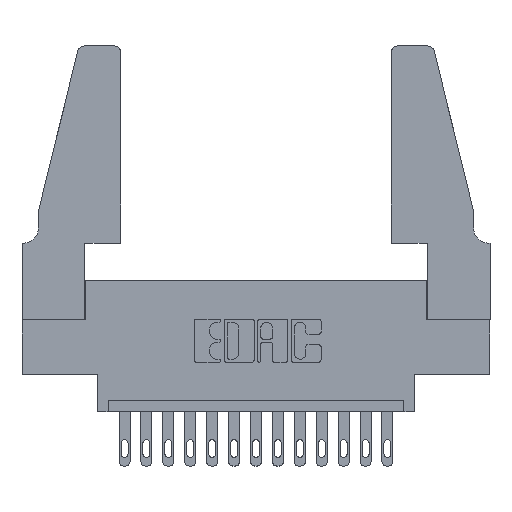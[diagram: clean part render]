
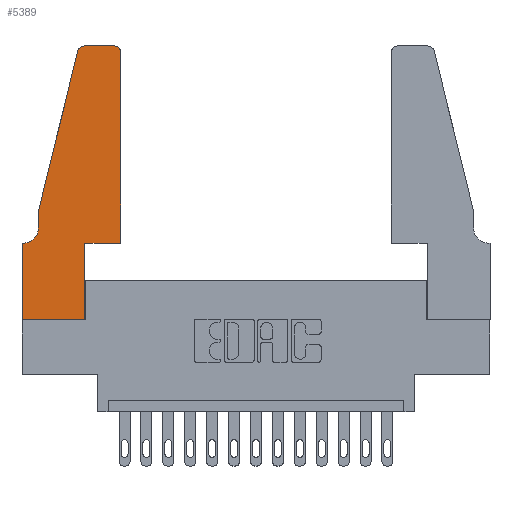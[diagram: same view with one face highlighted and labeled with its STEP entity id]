
A CAD part, top view. The second image highlights one B-rep face of the part: STEP entity #5389.
In plain terms, the highlighted planar face has unit normal (0, 0, 1).
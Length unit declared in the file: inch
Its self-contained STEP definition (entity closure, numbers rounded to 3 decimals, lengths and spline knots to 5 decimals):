
#267 = CARTESIAN_POINT ( 'NONE',  ( 0.2865, 0., 0.37 ) ) ;
#319 = DIRECTION ( 'NONE',  ( 0., 0., 1. ) ) ;
#414 = EDGE_CURVE ( 'NONE', #8223, #14759, #13134, .T. ) ;
#437 = DIRECTION ( 'NONE',  ( -1., 0., 0. ) ) ;
#600 = VECTOR ( 'NONE', #5861, 39.37008 ) ;
#714 = CARTESIAN_POINT ( 'NONE',  ( 0.284, 1.25, 0.37 ) ) ;
#724 = ORIENTED_EDGE ( 'NONE', *, *, #11421, .T. ) ;
#843 = AXIS2_PLACEMENT_3D ( 'NONE', #5069, #319, #2020 ) ;
#1082 = CARTESIAN_POINT ( 'NONE',  ( 0.0755, 0.42, 0.37 ) ) ;
#1410 = EDGE_CURVE ( 'NONE', #4058, #15772, #11135, .T. ) ;
#1481 = LINE ( 'NONE', #3548, #14192 ) ;
#1691 = AXIS2_PLACEMENT_3D ( 'NONE', #12727, #8869, #437 ) ;
#1774 = DIRECTION ( 'NONE',  ( 1., 0., 0. ) ) ;
#1813 = EDGE_CURVE ( 'NONE', #14759, #8313, #6549, .T. ) ;
#1819 = ORIENTED_EDGE ( 'NONE', *, *, #11017, .T. ) ;
#1976 = CARTESIAN_POINT ( 'NONE',  ( 0., 0., 0.37 ) ) ;
#2020 = DIRECTION ( 'NONE',  ( 1., 0., 0. ) ) ;
#2630 = CARTESIAN_POINT ( 'NONE',  ( 0., 0.35, 0.37 ) ) ;
#2651 = CARTESIAN_POINT ( 'NONE',  ( 0.0055, 0.35, 0.37 ) ) ;
#2877 = LINE ( 'NONE', #4622, #15357 ) ;
#2882 = CARTESIAN_POINT ( 'NONE',  ( 0.4505, 0.35, 0.37 ) ) ;
#2916 = DIRECTION ( 'NONE',  ( -1., 0., 0. ) ) ;
#2921 = VECTOR ( 'NONE', #13971, 39.37008 ) ;
#2950 = EDGE_CURVE ( 'NONE', #9746, #8223, #15342, .T. ) ;
#3084 = CARTESIAN_POINT ( 'NONE',  ( 0.0755, 0.5, 0.37 ) ) ;
#3548 = CARTESIAN_POINT ( 'NONE',  ( 0.0755, 0.35, 0.37 ) ) ;
#3623 = LINE ( 'NONE', #12809, #15502 ) ;
#3690 = LINE ( 'NONE', #6233, #2921 ) ;
#3698 = EDGE_CURVE ( 'NONE', #7521, #4464, #12444, .T. ) ;
#3913 = ORIENTED_EDGE ( 'NONE', *, *, #414, .T. ) ;
#4058 = VERTEX_POINT ( 'NONE', #6933 ) ;
#4184 = EDGE_CURVE ( 'NONE', #10795, #7521, #1481, .T. ) ;
#4200 = DIRECTION ( 'NONE',  ( -0.239, -0.971, 0. ) ) ;
#4308 = AXIS2_PLACEMENT_3D ( 'NONE', #13082, #5617, #1774 ) ;
#4347 = DIRECTION ( 'NONE',  ( 0., 0., 1. ) ) ;
#4464 = VERTEX_POINT ( 'NONE', #1976 ) ;
#4560 = ORIENTED_EDGE ( 'NONE', *, *, #1813, .T. ) ;
#4622 = CARTESIAN_POINT ( 'NONE',  ( 0.0755, 0.5, 0.37 ) ) ;
#4845 = CARTESIAN_POINT ( 'NONE',  ( 0.4205, 1.25, 0.37 ) ) ;
#4853 = ORIENTED_EDGE ( 'NONE', *, *, #3698, .T. ) ;
#5069 = CARTESIAN_POINT ( 'NONE',  ( 0.4205, 1.22, 0.37 ) ) ;
#5389 = ADVANCED_FACE ( 'NONE', ( #7193 ), #9322, .T. ) ;
#5466 = DIRECTION ( 'NONE',  ( 0., 1., 0. ) ) ;
#5472 = DIRECTION ( 'NONE',  ( 0., 1., 0. ) ) ;
#5617 = DIRECTION ( 'NONE',  ( 0., 0., 1. ) ) ;
#5827 = VECTOR ( 'NONE', #2916, 39.37008 ) ;
#5861 = DIRECTION ( 'NONE',  ( 1., 0., 0. ) ) ;
#6174 = AXIS2_PLACEMENT_3D ( 'NONE', #11691, #4347, #12932 ) ;
#6233 = CARTESIAN_POINT ( 'NONE',  ( 0., 0., 0.37 ) ) ;
#6360 = CARTESIAN_POINT ( 'NONE',  ( 0.0755, 0.5, 0.37 ) ) ;
#6549 = CIRCLE ( 'NONE', #6174, 0.03 ) ;
#6700 = ORIENTED_EDGE ( 'NONE', *, *, #13060, .T. ) ;
#6860 = ORIENTED_EDGE ( 'NONE', *, *, #2950, .T. ) ;
#6933 = CARTESIAN_POINT ( 'NONE',  ( 0.2865, 0.35, 0.37 ) ) ;
#7193 = FACE_OUTER_BOUND ( 'NONE', #8824, .T. ) ;
#7233 = DIRECTION ( 'NONE',  ( 0., -1., 0. ) ) ;
#7331 = CARTESIAN_POINT ( 'NONE',  ( 0.4505, 0.35, 0.37 ) ) ;
#7376 = VERTEX_POINT ( 'NONE', #1082 ) ;
#7521 = VERTEX_POINT ( 'NONE', #2630 ) ;
#7882 = EDGE_CURVE ( 'NONE', #13943, #7376, #2877, .T. ) ;
#8223 = VERTEX_POINT ( 'NONE', #4845 ) ;
#8303 = CARTESIAN_POINT ( 'NONE',  ( 0., 0., 0.37 ) ) ;
#8313 = VERTEX_POINT ( 'NONE', #13586 ) ;
#8824 = EDGE_LOOP ( 'NONE', ( #3913, #4560, #11824, #14111, #13491, #8832, #4853, #724, #1819, #14410, #6700, #6860 ) ) ;
#8832 = ORIENTED_EDGE ( 'NONE', *, *, #4184, .T. ) ;
#8869 = DIRECTION ( 'NONE',  ( 0., 0., -1. ) ) ;
#9322 = PLANE ( 'NONE',  #4308 ) ;
#9746 = VERTEX_POINT ( 'NONE', #11398 ) ;
#10795 = VERTEX_POINT ( 'NONE', #2651 ) ;
#10916 = EDGE_CURVE ( 'NONE', #8313, #13943, #15471, .T. ) ;
#11017 = EDGE_CURVE ( 'NONE', #15085, #4058, #3623, .T. ) ;
#11135 = LINE ( 'NONE', #12187, #600 ) ;
#11398 = CARTESIAN_POINT ( 'NONE',  ( 0.4505, 1.22, 0.37 ) ) ;
#11421 = EDGE_CURVE ( 'NONE', #4464, #15085, #3690, .T. ) ;
#11691 = CARTESIAN_POINT ( 'NONE',  ( 0.284, 1.22, 0.37 ) ) ;
#11824 = ORIENTED_EDGE ( 'NONE', *, *, #10916, .T. ) ;
#12121 = DIRECTION ( 'NONE',  ( -1., 0., 0. ) ) ;
#12187 = CARTESIAN_POINT ( 'NONE',  ( 0.4505, 0.35, 0.37 ) ) ;
#12202 = VECTOR ( 'NONE', #4200, 39.37008 ) ;
#12332 = EDGE_CURVE ( 'NONE', #7376, #10795, #14789, .T. ) ;
#12419 = VECTOR ( 'NONE', #13339, 39.37008 ) ;
#12444 = LINE ( 'NONE', #8303, #12419 ) ;
#12727 = CARTESIAN_POINT ( 'NONE',  ( 0.0055, 0.42, 0.37 ) ) ;
#12809 = CARTESIAN_POINT ( 'NONE',  ( 0.2865, 0.35, 0.37 ) ) ;
#12932 = DIRECTION ( 'NONE',  ( 1., 0., 0. ) ) ;
#13060 = EDGE_CURVE ( 'NONE', #15772, #9746, #15526, .T. ) ;
#13082 = CARTESIAN_POINT ( 'NONE',  ( 0., 0.35, 0.37 ) ) ;
#13134 = LINE ( 'NONE', #13548, #5827 ) ;
#13339 = DIRECTION ( 'NONE',  ( 0., -1., 0. ) ) ;
#13491 = ORIENTED_EDGE ( 'NONE', *, *, #12332, .T. ) ;
#13548 = CARTESIAN_POINT ( 'NONE',  ( 0.2605, 1.25, 0.37 ) ) ;
#13586 = CARTESIAN_POINT ( 'NONE',  ( 0.25487, 1.22718, 0.37 ) ) ;
#13943 = VERTEX_POINT ( 'NONE', #6360 ) ;
#13971 = DIRECTION ( 'NONE',  ( 1., 0., 0. ) ) ;
#14111 = ORIENTED_EDGE ( 'NONE', *, *, #7882, .T. ) ;
#14192 = VECTOR ( 'NONE', #12121, 39.37008 ) ;
#14410 = ORIENTED_EDGE ( 'NONE', *, *, #1410, .T. ) ;
#14759 = VERTEX_POINT ( 'NONE', #714 ) ;
#14789 = CIRCLE ( 'NONE', #1691, 0.07 ) ;
#15085 = VERTEX_POINT ( 'NONE', #267 ) ;
#15341 = VECTOR ( 'NONE', #5466, 39.37008 ) ;
#15342 = CIRCLE ( 'NONE', #843, 0.03 ) ;
#15357 = VECTOR ( 'NONE', #7233, 39.37008 ) ;
#15471 = LINE ( 'NONE', #3084, #12202 ) ;
#15502 = VECTOR ( 'NONE', #5472, 39.37008 ) ;
#15526 = LINE ( 'NONE', #2882, #15341 ) ;
#15772 = VERTEX_POINT ( 'NONE', #7331 ) ;
